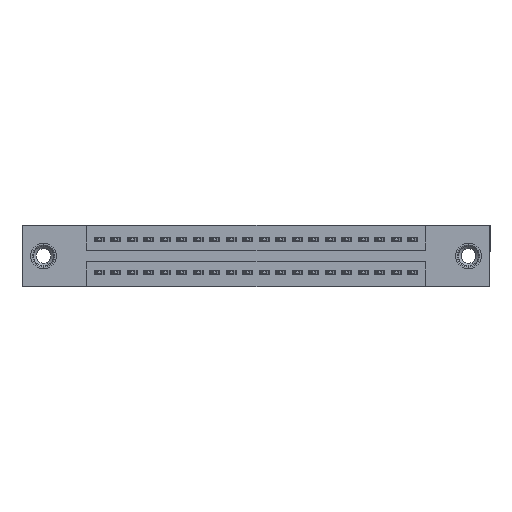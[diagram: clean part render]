
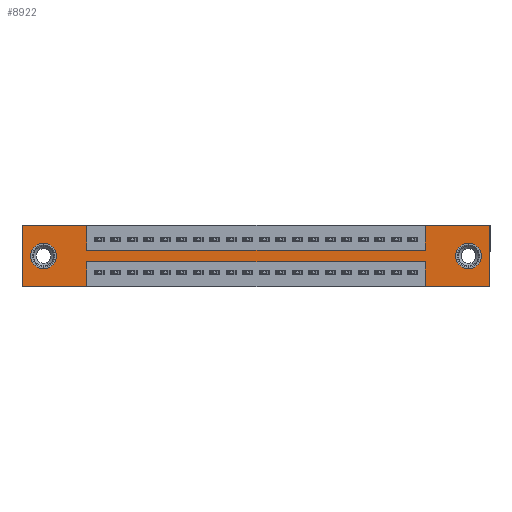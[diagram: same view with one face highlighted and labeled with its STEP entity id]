
A CAD part, front view. The second image highlights one B-rep face of the part: STEP entity #8922.
In plain terms, the highlighted planar face has unit normal (0, -1, 0).
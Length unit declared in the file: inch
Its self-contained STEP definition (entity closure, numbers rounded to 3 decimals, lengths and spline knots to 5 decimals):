
#39 = DIRECTION ( 'NONE',  ( 0., 0., 1. ) ) ;
#321 = EDGE_CURVE ( 'NONE', #17058, #14261, #6044, .T. ) ;
#860 = EDGE_CURVE ( 'NONE', #2053, #4374, #20401, .T. ) ;
#1124 = VERTEX_POINT ( 'NONE', #7132 ) ;
#1222 = ORIENTED_EDGE ( 'NONE', *, *, #11927, .F. ) ;
#1444 = DIRECTION ( 'NONE',  ( 0., 1., 0. ) ) ;
#1625 = ORIENTED_EDGE ( 'NONE', *, *, #10717, .F. ) ;
#1782 = VECTOR ( 'NONE', #16869, 39.37008 ) ;
#1848 = ORIENTED_EDGE ( 'NONE', *, *, #4644, .F. ) ;
#1943 = LINE ( 'NONE', #15874, #14503 ) ;
#1961 = FACE_OUTER_BOUND ( 'NONE', #14846, .T. ) ;
#2053 = VERTEX_POINT ( 'NONE', #13630 ) ;
#2294 = EDGE_CURVE ( 'NONE', #12609, #4223, #10487, .T. ) ;
#2297 = ORIENTED_EDGE ( 'NONE', *, *, #2294, .T. ) ;
#2416 = DIRECTION ( 'NONE',  ( 0., 0., 1. ) ) ;
#2619 = LINE ( 'NONE', #14892, #3856 ) ;
#2768 = DIRECTION ( 'NONE',  ( 0., 0., -1. ) ) ;
#2834 = EDGE_CURVE ( 'NONE', #13119, #12353, #1943, .T. ) ;
#2996 = EDGE_CURVE ( 'NONE', #4130, #15955, #11979, .T. ) ;
#3148 = DIRECTION ( 'NONE',  ( 0., 0., 1. ) ) ;
#3316 = ORIENTED_EDGE ( 'NONE', *, *, #860, .T. ) ;
#3372 = DIRECTION ( 'NONE',  ( 0., 1., 0. ) ) ;
#3451 = FACE_BOUND ( 'NONE', #16117, .T. ) ;
#3562 = DIRECTION ( 'NONE',  ( 1., 0., 0. ) ) ;
#3665 = VECTOR ( 'NONE', #15367, 39.37008 ) ;
#3785 = AXIS2_PLACEMENT_3D ( 'NONE', #16506, #9963, #17991 ) ;
#3856 = VECTOR ( 'NONE', #3562, 39.37008 ) ;
#3869 = VECTOR ( 'NONE', #16760, 39.37008 ) ;
#3904 = EDGE_CURVE ( 'NONE', #4374, #2053, #11420, .T. ) ;
#4051 = EDGE_CURVE ( 'NONE', #1124, #13119, #7664, .T. ) ;
#4130 = VERTEX_POINT ( 'NONE', #14615 ) ;
#4169 = DIRECTION ( 'NONE',  ( 0., 1., 0. ) ) ;
#4223 = VERTEX_POINT ( 'NONE', #11344 ) ;
#4291 = CARTESIAN_POINT ( 'NONE',  ( 0.3925, 0., -0.22 ) ) ;
#4374 = VERTEX_POINT ( 'NONE', #13939 ) ;
#4614 = CARTESIAN_POINT ( 'NONE',  ( 2.4425, 0., 0. ) ) ;
#4644 = EDGE_CURVE ( 'NONE', #20306, #4130, #20006, .T. ) ;
#4872 = CARTESIAN_POINT ( 'NONE',  ( 2.4425, 0., -0.15 ) ) ;
#5115 = VECTOR ( 'NONE', #17338, 39.37008 ) ;
#5167 = CARTESIAN_POINT ( 'NONE',  ( 0., 0., 0. ) ) ;
#5459 = FACE_BOUND ( 'NONE', #8259, .T. ) ;
#5524 = CARTESIAN_POINT ( 'NONE',  ( 2.835, 0., 0. ) ) ;
#5876 = VECTOR ( 'NONE', #3148, 39.37008 ) ;
#5992 = AXIS2_PLACEMENT_3D ( 'NONE', #11032, #1444, #7550 ) ;
#6044 = LINE ( 'NONE', #5524, #1782 ) ;
#6190 = CIRCLE ( 'NONE', #20366, 0.078 ) ;
#6241 = CARTESIAN_POINT ( 'NONE',  ( 2.705, 0., -0.185 ) ) ;
#7132 = CARTESIAN_POINT ( 'NONE',  ( 0., 0., -0.37 ) ) ;
#7155 = CARTESIAN_POINT ( 'NONE',  ( 0.3925, 0., -0.37 ) ) ;
#7355 = CARTESIAN_POINT ( 'NONE',  ( 2.705, 0., -0.185 ) ) ;
#7358 = ORIENTED_EDGE ( 'NONE', *, *, #20780, .T. ) ;
#7510 = VERTEX_POINT ( 'NONE', #10574 ) ;
#7550 = DIRECTION ( 'NONE',  ( 0., 0., 1. ) ) ;
#7592 = CARTESIAN_POINT ( 'NONE',  ( 0.3925, 0., 0. ) ) ;
#7664 = LINE ( 'NONE', #18868, #5876 ) ;
#7670 = AXIS2_PLACEMENT_3D ( 'NONE', #9789, #3372, #39 ) ;
#7694 = DIRECTION ( 'NONE',  ( 0., 0., 1. ) ) ;
#7860 = VECTOR ( 'NONE', #19784, 39.37008 ) ;
#7867 = DIRECTION ( 'NONE',  ( 1., 0., 0. ) ) ;
#8259 = EDGE_LOOP ( 'NONE', ( #17284, #3316 ) ) ;
#8661 = CARTESIAN_POINT ( 'NONE',  ( 2.835, 0., -0.37 ) ) ;
#8777 = CARTESIAN_POINT ( 'NONE',  ( 0.3925, 0., -0.22 ) ) ;
#8886 = VECTOR ( 'NONE', #2416, 39.37008 ) ;
#8922 = ADVANCED_FACE ( 'NONE', ( #3451, #5459, #1961 ), #10166, .T. ) ;
#9058 = VECTOR ( 'NONE', #13014, 39.37008 ) ;
#9090 = CARTESIAN_POINT ( 'NONE',  ( 2.4425, 0., 0. ) ) ;
#9094 = LINE ( 'NONE', #19498, #7860 ) ;
#9210 = DIRECTION ( 'NONE',  ( 0., 0., -1. ) ) ;
#9254 = LINE ( 'NONE', #9090, #18321 ) ;
#9485 = ORIENTED_EDGE ( 'NONE', *, *, #15253, .F. ) ;
#9658 = ORIENTED_EDGE ( 'NONE', *, *, #321, .F. ) ;
#9789 = CARTESIAN_POINT ( 'NONE',  ( 0.13, 0., -0.185 ) ) ;
#9873 = CARTESIAN_POINT ( 'NONE',  ( 2.705, 0., -0.107 ) ) ;
#9940 = CARTESIAN_POINT ( 'NONE',  ( 0., 0., -0.37 ) ) ;
#9963 = DIRECTION ( 'NONE',  ( 0., -1., 0. ) ) ;
#10166 = PLANE ( 'NONE',  #3785 ) ;
#10401 = CARTESIAN_POINT ( 'NONE',  ( 2.835, 0., 0. ) ) ;
#10431 = LINE ( 'NONE', #18904, #5115 ) ;
#10487 = CIRCLE ( 'NONE', #12091, 0.078 ) ;
#10574 = CARTESIAN_POINT ( 'NONE',  ( 0.3925, 0., -0.15 ) ) ;
#10717 = EDGE_CURVE ( 'NONE', #14261, #20306, #10925, .T. ) ;
#10925 = LINE ( 'NONE', #9940, #3869 ) ;
#11032 = CARTESIAN_POINT ( 'NONE',  ( 0.13, 0., -0.185 ) ) ;
#11139 = EDGE_CURVE ( 'NONE', #15463, #1124, #10431, .T. ) ;
#11344 = CARTESIAN_POINT ( 'NONE',  ( 2.705, 0., -0.263 ) ) ;
#11420 = CIRCLE ( 'NONE', #7670, 0.078 ) ;
#11638 = EDGE_CURVE ( 'NONE', #12555, #17058, #2619, .T. ) ;
#11876 = ORIENTED_EDGE ( 'NONE', *, *, #19568, .F. ) ;
#11927 = EDGE_CURVE ( 'NONE', #7510, #18580, #18212, .T. ) ;
#11979 = LINE ( 'NONE', #8777, #3665 ) ;
#12091 = AXIS2_PLACEMENT_3D ( 'NONE', #6241, #17492, #9210 ) ;
#12102 = CARTESIAN_POINT ( 'NONE',  ( 0.3925, 0., -0.15 ) ) ;
#12353 = VERTEX_POINT ( 'NONE', #7592 ) ;
#12555 = VERTEX_POINT ( 'NONE', #4614 ) ;
#12609 = VERTEX_POINT ( 'NONE', #9873 ) ;
#12854 = ORIENTED_EDGE ( 'NONE', *, *, #16230, .F. ) ;
#13014 = DIRECTION ( 'NONE',  ( 0., 0., -1. ) ) ;
#13119 = VERTEX_POINT ( 'NONE', #5167 ) ;
#13299 = ORIENTED_EDGE ( 'NONE', *, *, #2834, .F. ) ;
#13305 = LINE ( 'NONE', #19583, #9058 ) ;
#13630 = CARTESIAN_POINT ( 'NONE',  ( 0.13, 0., -0.263 ) ) ;
#13926 = VECTOR ( 'NONE', #20370, 39.37008 ) ;
#13939 = CARTESIAN_POINT ( 'NONE',  ( 0.13, 0., -0.107 ) ) ;
#14115 = CARTESIAN_POINT ( 'NONE',  ( 2.4425, 0., -0.37 ) ) ;
#14261 = VERTEX_POINT ( 'NONE', #8661 ) ;
#14503 = VECTOR ( 'NONE', #7867, 39.37008 ) ;
#14615 = CARTESIAN_POINT ( 'NONE',  ( 2.4425, 0., -0.22 ) ) ;
#14846 = EDGE_LOOP ( 'NONE', ( #9485, #17755, #1848, #1625, #9658, #20323, #11876, #1222, #12854, #13299, #20070, #17391 ) ) ;
#14892 = CARTESIAN_POINT ( 'NONE',  ( 0., 0., 0. ) ) ;
#15253 = EDGE_CURVE ( 'NONE', #15955, #15463, #9094, .T. ) ;
#15367 = DIRECTION ( 'NONE',  ( -1., 0., 0. ) ) ;
#15463 = VERTEX_POINT ( 'NONE', #7155 ) ;
#15874 = CARTESIAN_POINT ( 'NONE',  ( 0., 0., 0. ) ) ;
#15955 = VERTEX_POINT ( 'NONE', #4291 ) ;
#16117 = EDGE_LOOP ( 'NONE', ( #2297, #7358 ) ) ;
#16230 = EDGE_CURVE ( 'NONE', #12353, #7510, #13305, .T. ) ;
#16506 = CARTESIAN_POINT ( 'NONE',  ( 0., 0., -0.37 ) ) ;
#16760 = DIRECTION ( 'NONE',  ( -1., 0., 0. ) ) ;
#16869 = DIRECTION ( 'NONE',  ( 0., 0., -1. ) ) ;
#17058 = VERTEX_POINT ( 'NONE', #10401 ) ;
#17284 = ORIENTED_EDGE ( 'NONE', *, *, #3904, .T. ) ;
#17338 = DIRECTION ( 'NONE',  ( -1., 0., 0. ) ) ;
#17391 = ORIENTED_EDGE ( 'NONE', *, *, #11139, .F. ) ;
#17492 = DIRECTION ( 'NONE',  ( 0., 1., 0. ) ) ;
#17755 = ORIENTED_EDGE ( 'NONE', *, *, #2996, .F. ) ;
#17991 = DIRECTION ( 'NONE',  ( 0., 0., -1. ) ) ;
#18212 = LINE ( 'NONE', #12102, #13926 ) ;
#18321 = VECTOR ( 'NONE', #7694, 39.37008 ) ;
#18580 = VERTEX_POINT ( 'NONE', #4872 ) ;
#18868 = CARTESIAN_POINT ( 'NONE',  ( 0., 0., 0. ) ) ;
#18904 = CARTESIAN_POINT ( 'NONE',  ( 0., 0., -0.37 ) ) ;
#18963 = CARTESIAN_POINT ( 'NONE',  ( 2.4425, 0., -0.37 ) ) ;
#19498 = CARTESIAN_POINT ( 'NONE',  ( 0.3925, 0., -0.37 ) ) ;
#19568 = EDGE_CURVE ( 'NONE', #18580, #12555, #9254, .T. ) ;
#19583 = CARTESIAN_POINT ( 'NONE',  ( 0.3925, 0., 0. ) ) ;
#19784 = DIRECTION ( 'NONE',  ( 0., 0., -1. ) ) ;
#20006 = LINE ( 'NONE', #18963, #8886 ) ;
#20070 = ORIENTED_EDGE ( 'NONE', *, *, #4051, .F. ) ;
#20306 = VERTEX_POINT ( 'NONE', #14115 ) ;
#20323 = ORIENTED_EDGE ( 'NONE', *, *, #11638, .F. ) ;
#20366 = AXIS2_PLACEMENT_3D ( 'NONE', #7355, #4169, #2768 ) ;
#20370 = DIRECTION ( 'NONE',  ( 1., 0., 0. ) ) ;
#20401 = CIRCLE ( 'NONE', #5992, 0.078 ) ;
#20780 = EDGE_CURVE ( 'NONE', #4223, #12609, #6190, .T. ) ;
